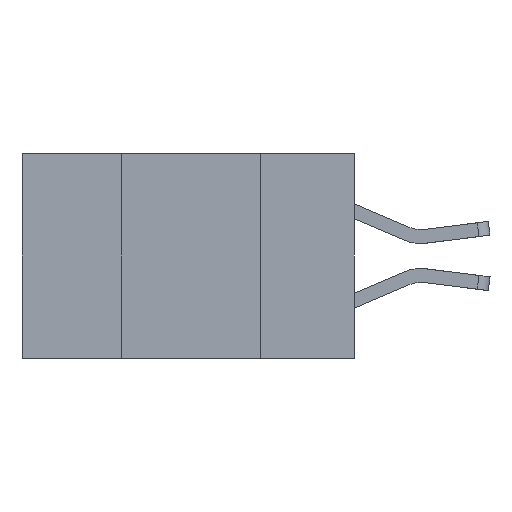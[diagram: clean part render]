
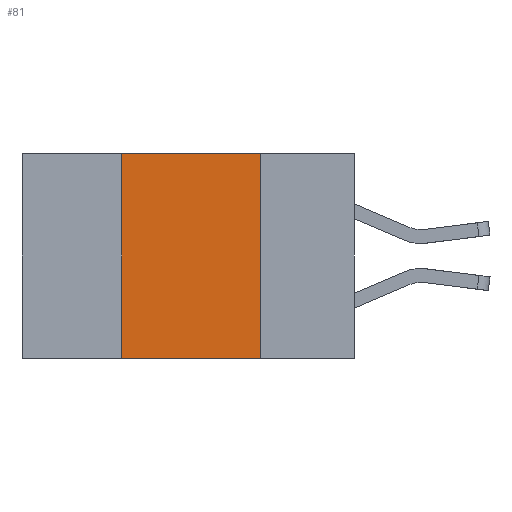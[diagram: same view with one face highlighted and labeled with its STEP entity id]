
A CAD part, left-side view. The second image highlights one B-rep face of the part: STEP entity #81.
In plain terms, the highlighted planar face has unit normal (-1, 0, 0).
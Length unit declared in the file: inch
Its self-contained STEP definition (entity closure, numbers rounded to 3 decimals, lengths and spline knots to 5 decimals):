
#81 = ADVANCED_FACE ( 'NONE', ( #3321 ), #471, .F. ) ;
#113 = VECTOR ( 'NONE', #8014, 39.37008 ) ;
#471 = PLANE ( 'NONE',  #786 ) ;
#544 = ORIENTED_EDGE ( 'NONE', *, *, #2020, .F. ) ;
#670 = LINE ( 'NONE', #5970, #4813 ) ;
#772 = CARTESIAN_POINT ( 'NONE',  ( 0., 0.42, 0. ) ) ;
#786 = AXIS2_PLACEMENT_3D ( 'NONE', #4697, #7822, #4547 ) ;
#959 = VERTEX_POINT ( 'NONE', #8948 ) ;
#1133 = CARTESIAN_POINT ( 'NONE',  ( 0., 0.17, -0.37 ) ) ;
#2020 = EDGE_CURVE ( 'NONE', #959, #7537, #5042, .T. ) ;
#2021 = EDGE_CURVE ( 'NONE', #5067, #959, #670, .T. ) ;
#2024 = EDGE_CURVE ( 'NONE', #2781, #5067, #8234, .T. ) ;
#2035 = EDGE_CURVE ( 'NONE', #2781, #7537, #2481, .T. ) ;
#2481 = LINE ( 'NONE', #2777, #113 ) ;
#2504 = CARTESIAN_POINT ( 'NONE',  ( 0., 0.42, -0.37 ) ) ;
#2777 = CARTESIAN_POINT ( 'NONE',  ( 0., 0.6, -0.37 ) ) ;
#2781 = VERTEX_POINT ( 'NONE', #2504 ) ;
#3321 = FACE_OUTER_BOUND ( 'NONE', #5153, .T. ) ;
#4531 = ORIENTED_EDGE ( 'NONE', *, *, #2024, .F. ) ;
#4547 = DIRECTION ( 'NONE',  ( 0., 0., -1. ) ) ;
#4697 = CARTESIAN_POINT ( 'NONE',  ( 0., 0.6, 0. ) ) ;
#4776 = DIRECTION ( 'NONE',  ( 0., -1., 0. ) ) ;
#4813 = VECTOR ( 'NONE', #4776, 39.37008 ) ;
#4927 = DIRECTION ( 'NONE',  ( 0., 0., 1. ) ) ;
#5004 = CARTESIAN_POINT ( 'NONE',  ( 0., 0.42, -0.37 ) ) ;
#5042 = LINE ( 'NONE', #8549, #8433 ) ;
#5067 = VERTEX_POINT ( 'NONE', #772 ) ;
#5153 = EDGE_LOOP ( 'NONE', ( #544, #9294, #4531, #5284 ) ) ;
#5284 = ORIENTED_EDGE ( 'NONE', *, *, #2035, .T. ) ;
#5970 = CARTESIAN_POINT ( 'NONE',  ( 0., 0.6, 0. ) ) ;
#6793 = VECTOR ( 'NONE', #4927, 39.37008 ) ;
#7537 = VERTEX_POINT ( 'NONE', #1133 ) ;
#7822 = DIRECTION ( 'NONE',  ( 1., 0., 0. ) ) ;
#7869 = DIRECTION ( 'NONE',  ( 0., 0., -1. ) ) ;
#8014 = DIRECTION ( 'NONE',  ( 0., -1., 0. ) ) ;
#8234 = LINE ( 'NONE', #5004, #6793 ) ;
#8433 = VECTOR ( 'NONE', #7869, 39.37008 ) ;
#8549 = CARTESIAN_POINT ( 'NONE',  ( 0., 0.17, -0.37 ) ) ;
#8948 = CARTESIAN_POINT ( 'NONE',  ( 0., 0.17, 0. ) ) ;
#9294 = ORIENTED_EDGE ( 'NONE', *, *, #2021, .F. ) ;
